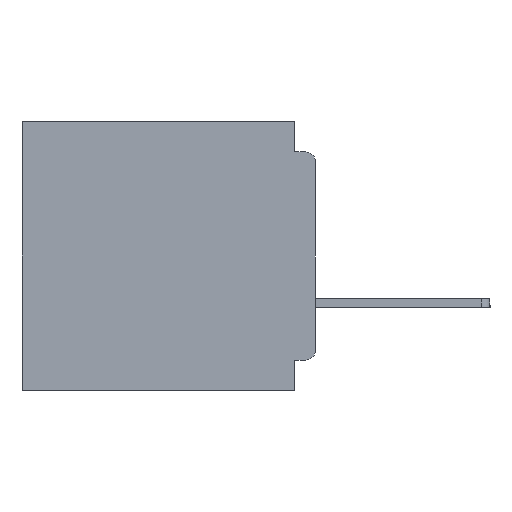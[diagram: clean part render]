
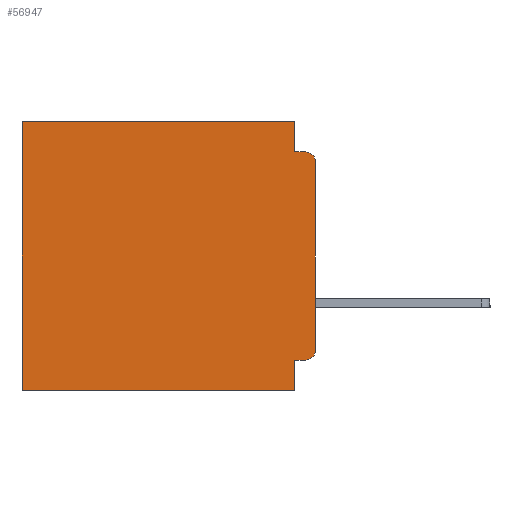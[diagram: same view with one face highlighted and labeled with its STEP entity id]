
A CAD part, left-side view. The second image highlights one B-rep face of the part: STEP entity #56947.
In plain terms, the highlighted planar face has unit normal (-1, 0, 0).
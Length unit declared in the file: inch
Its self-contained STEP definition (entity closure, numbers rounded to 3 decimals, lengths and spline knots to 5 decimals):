
#45 = CARTESIAN_POINT ( 'NONE',  ( 0.3, 0.015, -0.34 ) ) ;
#263 = EDGE_CURVE ( 'NONE', #50718, #47008, #38858, .T. ) ;
#333 = EDGE_CURVE ( 'NONE', #50718, #53920, #60133, .T. ) ;
#745 = VECTOR ( 'NONE', #55219, 39.37008 ) ;
#788 = CARTESIAN_POINT ( 'NONE',  ( 0.3, 0.015, -0.045 ) ) ;
#790 = VERTEX_POINT ( 'NONE', #55854 ) ;
#2071 = LINE ( 'NONE', #52524, #28569 ) ;
#3243 = CARTESIAN_POINT ( 'NONE',  ( 0.3, 0.031, 0. ) ) ;
#3413 = DIRECTION ( 'NONE',  ( 0., 0., -1. ) ) ;
#4649 = DIRECTION ( 'NONE',  ( -1., 0., 0. ) ) ;
#4962 = EDGE_CURVE ( 'NONE', #47008, #11313, #2071, .T. ) ;
#5177 = DIRECTION ( 'NONE',  ( 0., 0., -1. ) ) ;
#5929 = ORIENTED_EDGE ( 'NONE', *, *, #17075, .F. ) ;
#6174 = CIRCLE ( 'NONE', #19654, 0.015 ) ;
#6842 = CARTESIAN_POINT ( 'NONE',  ( 0.3, 0., -0.06 ) ) ;
#7433 = CARTESIAN_POINT ( 'NONE',  ( 0.3, 0., -0.4 ) ) ;
#7879 = VECTOR ( 'NONE', #19821, 39.37008 ) ;
#9483 = EDGE_CURVE ( 'NONE', #40862, #790, #54794, .T. ) ;
#10259 = LINE ( 'NONE', #25626, #48124 ) ;
#10460 = ORIENTED_EDGE ( 'NONE', *, *, #57127, .F. ) ;
#11106 = ORIENTED_EDGE ( 'NONE', *, *, #59791, .T. ) ;
#11313 = VERTEX_POINT ( 'NONE', #788 ) ;
#13597 = CARTESIAN_POINT ( 'NONE',  ( 0.3, 0.437, 0. ) ) ;
#13979 = CARTESIAN_POINT ( 'NONE',  ( 0.3, 0.031, -0.4 ) ) ;
#15868 = CARTESIAN_POINT ( 'NONE',  ( 0.3, 0., -0.355 ) ) ;
#16939 = CARTESIAN_POINT ( 'NONE',  ( 0.3, 0.031, -0.4 ) ) ;
#17075 = EDGE_CURVE ( 'NONE', #43038, #22277, #53449, .T. ) ;
#17206 = ORIENTED_EDGE ( 'NONE', *, *, #4962, .F. ) ;
#18037 = EDGE_CURVE ( 'NONE', #40862, #11313, #6174, .T. ) ;
#18831 = EDGE_LOOP ( 'NONE', ( #37305, #39879, #17206, #52716, #31209, #11106, #21625, #10460, #5929, #55941 ) ) ;
#19654 = AXIS2_PLACEMENT_3D ( 'NONE', #34327, #4649, #39275 ) ;
#19814 = CARTESIAN_POINT ( 'NONE',  ( 0.3, 0., 0. ) ) ;
#19821 = DIRECTION ( 'NONE',  ( 0., 1., 0. ) ) ;
#20924 = VERTEX_POINT ( 'NONE', #16939 ) ;
#21625 = ORIENTED_EDGE ( 'NONE', *, *, #44389, .F. ) ;
#22277 = VERTEX_POINT ( 'NONE', #45825 ) ;
#22481 = FACE_OUTER_BOUND ( 'NONE', #18831, .T. ) ;
#23009 = DIRECTION ( 'NONE',  ( 0., -1., 0. ) ) ;
#23384 = CARTESIAN_POINT ( 'NONE',  ( 0.3, 0.015, -0.355 ) ) ;
#25070 = VECTOR ( 'NONE', #49093, 39.37008 ) ;
#25284 = AXIS2_PLACEMENT_3D ( 'NONE', #7433, #61535, #32355 ) ;
#25626 = CARTESIAN_POINT ( 'NONE',  ( 0.3, 0.437, -0.4 ) ) ;
#26622 = LINE ( 'NONE', #29302, #25070 ) ;
#28139 = CIRCLE ( 'NONE', #36724, 0.015 ) ;
#28569 = VECTOR ( 'NONE', #23009, 39.37008 ) ;
#29302 = CARTESIAN_POINT ( 'NONE',  ( 0.3, 0., -0.4 ) ) ;
#31209 = ORIENTED_EDGE ( 'NONE', *, *, #333, .T. ) ;
#32355 = DIRECTION ( 'NONE',  ( 0., 0., -1. ) ) ;
#32722 = CARTESIAN_POINT ( 'NONE',  ( 0.3, 0.437, -0.4 ) ) ;
#34327 = CARTESIAN_POINT ( 'NONE',  ( 0.3, 0.015, -0.06 ) ) ;
#34837 = DIRECTION ( 'NONE',  ( -1., 0., 0. ) ) ;
#36341 = LINE ( 'NONE', #13979, #60748 ) ;
#36512 = EDGE_CURVE ( 'NONE', #43038, #790, #28139, .T. ) ;
#36724 = AXIS2_PLACEMENT_3D ( 'NONE', #45, #34837, #5177 ) ;
#37305 = ORIENTED_EDGE ( 'NONE', *, *, #9483, .F. ) ;
#38858 = LINE ( 'NONE', #3243, #50436 ) ;
#39275 = DIRECTION ( 'NONE',  ( 0., 0., -1. ) ) ;
#39879 = ORIENTED_EDGE ( 'NONE', *, *, #18037, .T. ) ;
#40862 = VERTEX_POINT ( 'NONE', #6842 ) ;
#43038 = VERTEX_POINT ( 'NONE', #23384 ) ;
#44389 = EDGE_CURVE ( 'NONE', #20924, #60072, #26622, .T. ) ;
#45825 = CARTESIAN_POINT ( 'NONE',  ( 0.3, 0.031, -0.355 ) ) ;
#47008 = VERTEX_POINT ( 'NONE', #49651 ) ;
#48124 = VECTOR ( 'NONE', #50221, 39.37008 ) ;
#49093 = DIRECTION ( 'NONE',  ( 0., 1., 0. ) ) ;
#49651 = CARTESIAN_POINT ( 'NONE',  ( 0.3, 0.031, -0.045 ) ) ;
#50221 = DIRECTION ( 'NONE',  ( 0., 0., -1. ) ) ;
#50436 = VECTOR ( 'NONE', #3413, 39.37008 ) ;
#50718 = VERTEX_POINT ( 'NONE', #60236 ) ;
#52524 = CARTESIAN_POINT ( 'NONE',  ( 0.3, 0., -0.045 ) ) ;
#52716 = ORIENTED_EDGE ( 'NONE', *, *, #263, .F. ) ;
#53102 = CARTESIAN_POINT ( 'NONE',  ( 0.3, 0., -0.4 ) ) ;
#53296 = VECTOR ( 'NONE', #57900, 39.37008 ) ;
#53449 = LINE ( 'NONE', #15868, #745 ) ;
#53920 = VERTEX_POINT ( 'NONE', #13597 ) ;
#54794 = LINE ( 'NONE', #53102, #53296 ) ;
#55219 = DIRECTION ( 'NONE',  ( 0., 1., 0. ) ) ;
#55854 = CARTESIAN_POINT ( 'NONE',  ( 0.3, 0., -0.34 ) ) ;
#55941 = ORIENTED_EDGE ( 'NONE', *, *, #36512, .T. ) ;
#56723 = PLANE ( 'NONE',  #25284 ) ;
#56947 = ADVANCED_FACE ( 'NONE', ( #22481 ), #56723, .F. ) ;
#57127 = EDGE_CURVE ( 'NONE', #22277, #20924, #36341, .T. ) ;
#57900 = DIRECTION ( 'NONE',  ( 0., 0., -1. ) ) ;
#59791 = EDGE_CURVE ( 'NONE', #53920, #60072, #10259, .T. ) ;
#60072 = VERTEX_POINT ( 'NONE', #32722 ) ;
#60133 = LINE ( 'NONE', #19814, #7879 ) ;
#60236 = CARTESIAN_POINT ( 'NONE',  ( 0.3, 0.031, 0. ) ) ;
#60748 = VECTOR ( 'NONE', #62970, 39.37008 ) ;
#61535 = DIRECTION ( 'NONE',  ( 1., 0., 0. ) ) ;
#62970 = DIRECTION ( 'NONE',  ( 0., 0., -1. ) ) ;
